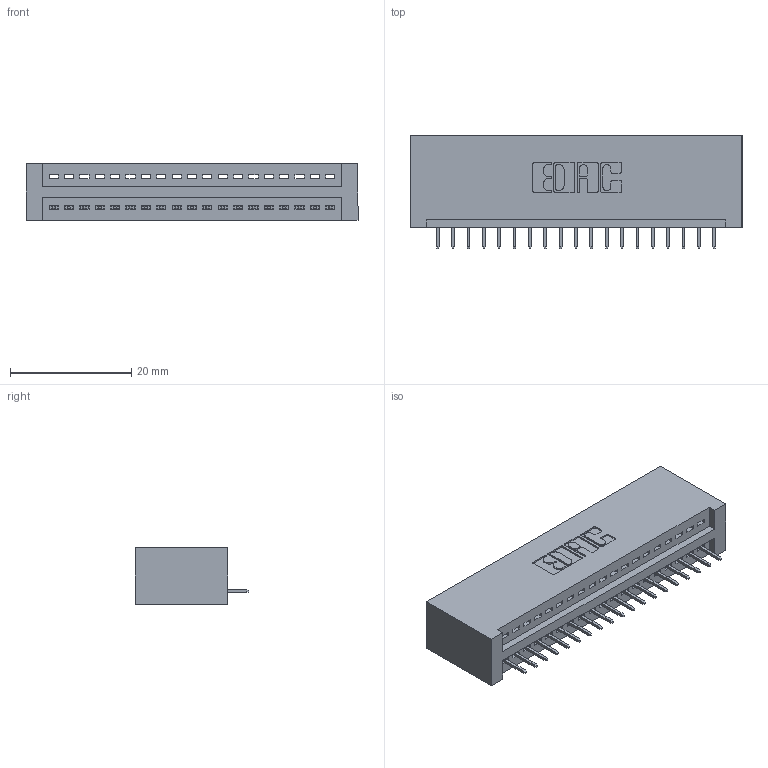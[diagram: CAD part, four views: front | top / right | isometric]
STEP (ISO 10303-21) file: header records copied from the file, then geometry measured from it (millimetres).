
FILE_DESCRIPTION (( 'STEP AP203' ), '1' );
FILE_NAME ('895-019-525-101.STEP', '2020-09-25T07:16:04', ( '' ), ( '' ), 'SwSTEP 2.0', 'SolidWorks 2020', '' );
FILE_SCHEMA (( 'CONFIG_CONTROL_DESIGN' ));
Length unit declared in the file: inch
Products named in the file (3): 895-019-525-101; 845 Part_No Mounting Lugs; 345-292-001_345-293-125
Assembly tree (20 placements, depth 2):
  895-019-525-101
    845 Part_No Mounting Lugs
    345-292-001_345-293-125  x19
Bounding box: 54.86 x 18.72 x 9.4 mm (x, y, z)
Volume: 5529.4 mm3; surface area: 6966.9 mm2
Topology: 20 solids, 20 shells, 1296 faces, 3737 edges, 2414 vertices
Faces by surface type: plane 950, cylinder 346
Entity records: 17193 total; most frequent: CARTESIAN_POINT 2985, ORIENTED_EDGE 2938, DIRECTION 2635, EDGE_CURVE 1469, VECTOR 1273, LINE 1273, VERTEX_POINT 974, AXIS2_PLACEMENT_3D 681
